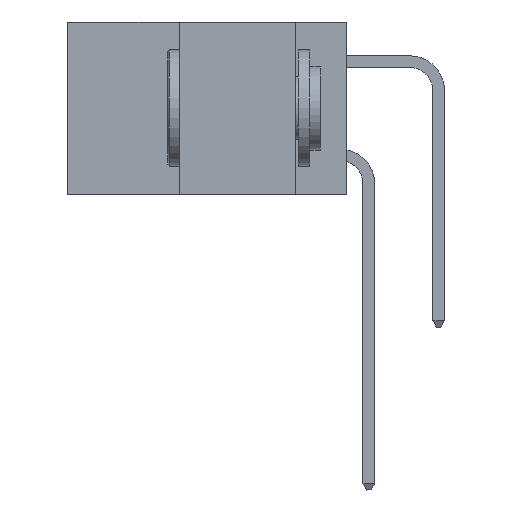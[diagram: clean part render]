
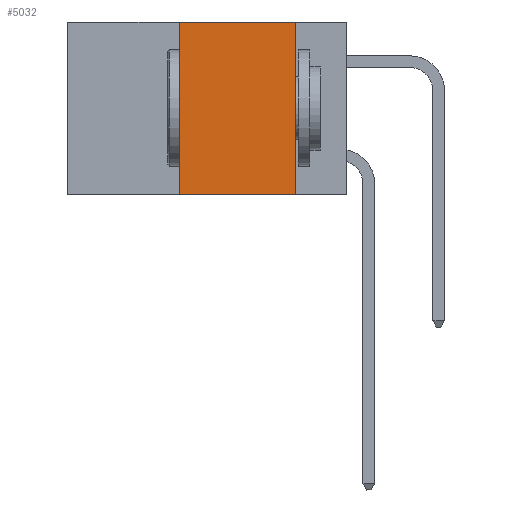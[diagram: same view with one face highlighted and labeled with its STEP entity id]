
A CAD part, left-side view. The second image highlights one B-rep face of the part: STEP entity #5032.
In plain terms, the highlighted planar face has unit normal (-1, 0, 0).
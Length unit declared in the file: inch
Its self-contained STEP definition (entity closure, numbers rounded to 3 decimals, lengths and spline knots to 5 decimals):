
#4702 = EDGE_CURVE ( 'NONE', #42745, #20664, #10459, .T. ) ;
#5032 = ADVANCED_FACE ( 'NONE', ( #36395 ), #9486, .F. ) ;
#6995 = DIRECTION ( 'NONE',  ( 0., -1., 0. ) ) ;
#8512 = ORIENTED_EDGE ( 'NONE', *, *, #10153, .F. ) ;
#9486 = PLANE ( 'NONE',  #15564 ) ;
#10153 = EDGE_CURVE ( 'NONE', #37306, #35755, #21501, .T. ) ;
#10194 = CARTESIAN_POINT ( 'NONE',  ( 0., 0.11, 0. ) ) ;
#10459 = LINE ( 'NONE', #23429, #20134 ) ;
#11682 = VECTOR ( 'NONE', #51489, 39.37008 ) ;
#13097 = VECTOR ( 'NONE', #44492, 39.37008 ) ;
#15564 = AXIS2_PLACEMENT_3D ( 'NONE', #25570, #25760, #46627 ) ;
#15780 = CARTESIAN_POINT ( 'NONE',  ( 0., 0.36, 0. ) ) ;
#20134 = VECTOR ( 'NONE', #6995, 39.37008 ) ;
#20664 = VERTEX_POINT ( 'NONE', #38530 ) ;
#20807 = ORIENTED_EDGE ( 'NONE', *, *, #25378, .F. ) ;
#21501 = LINE ( 'NONE', #41037, #13097 ) ;
#22682 = EDGE_CURVE ( 'NONE', #42745, #37306, #41290, .T. ) ;
#23092 = CARTESIAN_POINT ( 'NONE',  ( 0., 0.36, 0. ) ) ;
#23429 = CARTESIAN_POINT ( 'NONE',  ( 0., 0.6, -0.37 ) ) ;
#23798 = ORIENTED_EDGE ( 'NONE', *, *, #22682, .F. ) ;
#25378 = EDGE_CURVE ( 'NONE', #35755, #20664, #36986, .T. ) ;
#25570 = CARTESIAN_POINT ( 'NONE',  ( 0., 0.6, 0. ) ) ;
#25760 = DIRECTION ( 'NONE',  ( 1., 0., 0. ) ) ;
#28715 = CARTESIAN_POINT ( 'NONE',  ( 0., 0.36, -0.37 ) ) ;
#29558 = VECTOR ( 'NONE', #39624, 39.37008 ) ;
#35212 = CARTESIAN_POINT ( 'NONE',  ( 0., 0.11, 0. ) ) ;
#35755 = VERTEX_POINT ( 'NONE', #10194 ) ;
#36395 = FACE_OUTER_BOUND ( 'NONE', #39906, .T. ) ;
#36498 = ORIENTED_EDGE ( 'NONE', *, *, #4702, .T. ) ;
#36986 = LINE ( 'NONE', #35212, #11682 ) ;
#37306 = VERTEX_POINT ( 'NONE', #15780 ) ;
#38530 = CARTESIAN_POINT ( 'NONE',  ( 0., 0.11, -0.37 ) ) ;
#39624 = DIRECTION ( 'NONE',  ( 0., 0., 1. ) ) ;
#39906 = EDGE_LOOP ( 'NONE', ( #20807, #8512, #23798, #36498 ) ) ;
#41037 = CARTESIAN_POINT ( 'NONE',  ( 0., 0.6, 0. ) ) ;
#41290 = LINE ( 'NONE', #23092, #29558 ) ;
#42745 = VERTEX_POINT ( 'NONE', #28715 ) ;
#44492 = DIRECTION ( 'NONE',  ( 0., -1., 0. ) ) ;
#46627 = DIRECTION ( 'NONE',  ( 0., 0., -1. ) ) ;
#51489 = DIRECTION ( 'NONE',  ( 0., 0., -1. ) ) ;
